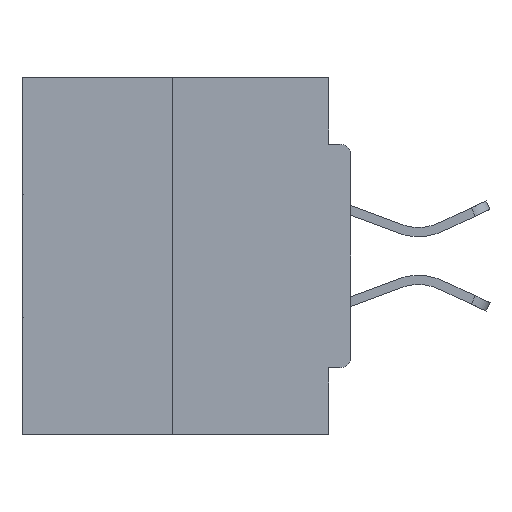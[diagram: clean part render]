
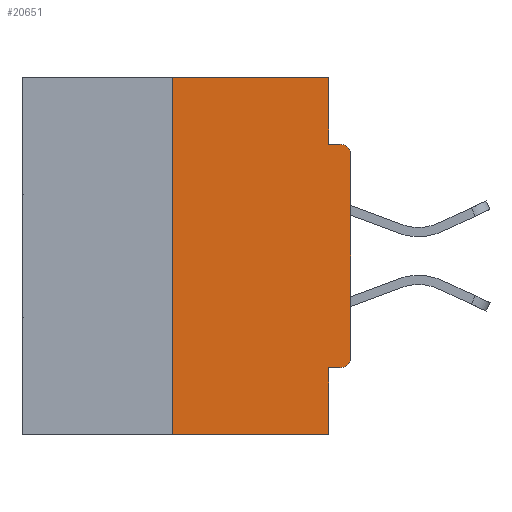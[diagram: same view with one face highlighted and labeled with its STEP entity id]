
A CAD part, left-side view. The second image highlights one B-rep face of the part: STEP entity #20651.
In plain terms, the highlighted planar face has unit normal (-1, 0, 0).
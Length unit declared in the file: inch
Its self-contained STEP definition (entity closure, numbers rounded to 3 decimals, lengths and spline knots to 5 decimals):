
#1036 = CARTESIAN_POINT ( 'NONE',  ( 0., 0., -0.0935 ) ) ;
#1229 = VERTEX_POINT ( 'NONE', #34514 ) ;
#1658 = VECTOR ( 'NONE', #26369, 39.37008 ) ;
#1724 = VECTOR ( 'NONE', #2325, 39.37008 ) ;
#2126 = ORIENTED_EDGE ( 'NONE', *, *, #22680, .F. ) ;
#2325 = DIRECTION ( 'NONE',  ( 0., 0., 1. ) ) ;
#2469 = EDGE_CURVE ( 'NONE', #12966, #9747, #3826, .T. ) ;
#2650 = PLANE ( 'NONE',  #9495 ) ;
#3304 = VERTEX_POINT ( 'NONE', #9077 ) ;
#3761 = CARTESIAN_POINT ( 'NONE',  ( 0., 0.031, -0.4065 ) ) ;
#3826 = LINE ( 'NONE', #34916, #12984 ) ;
#4241 = ORIENTED_EDGE ( 'NONE', *, *, #29061, .F. ) ;
#4413 = DIRECTION ( 'NONE',  ( 0., -1., 0. ) ) ;
#5447 = DIRECTION ( 'NONE',  ( 0., 0., -1. ) ) ;
#5550 = ORIENTED_EDGE ( 'NONE', *, *, #33950, .F. ) ;
#5840 = DIRECTION ( 'NONE',  ( 0., 0., -1. ) ) ;
#8347 = VECTOR ( 'NONE', #35288, 39.37008 ) ;
#8620 = CARTESIAN_POINT ( 'NONE',  ( 0., 0.46, 0. ) ) ;
#9013 = DIRECTION ( 'NONE',  ( 1., 0., 0. ) ) ;
#9077 = CARTESIAN_POINT ( 'NONE',  ( 0., 0.25, 0. ) ) ;
#9121 = ORIENTED_EDGE ( 'NONE', *, *, #2469, .T. ) ;
#9495 = AXIS2_PLACEMENT_3D ( 'NONE', #8620, #9013, #5447 ) ;
#9653 = VECTOR ( 'NONE', #19865, 39.37008 ) ;
#9747 = VERTEX_POINT ( 'NONE', #37930 ) ;
#10101 = DIRECTION ( 'NONE',  ( 0., -1., 0. ) ) ;
#10767 = CIRCLE ( 'NONE', #20283, 0.015 ) ;
#11812 = DIRECTION ( 'NONE',  ( -1., 0., 0. ) ) ;
#12966 = VERTEX_POINT ( 'NONE', #30072 ) ;
#12984 = VECTOR ( 'NONE', #4413, 39.37008 ) ;
#13275 = EDGE_CURVE ( 'NONE', #37519, #1229, #38341, .T. ) ;
#13367 = EDGE_CURVE ( 'NONE', #35274, #18704, #17462, .T. ) ;
#14390 = EDGE_CURVE ( 'NONE', #3304, #25434, #18477, .T. ) ;
#14423 = CARTESIAN_POINT ( 'NONE',  ( 0., 0.031, -0.5 ) ) ;
#14607 = VECTOR ( 'NONE', #37385, 39.37008 ) ;
#14666 = LINE ( 'NONE', #26224, #1724 ) ;
#15212 = CARTESIAN_POINT ( 'NONE',  ( 0., 0., -0.3915 ) ) ;
#15776 = EDGE_CURVE ( 'NONE', #27937, #37519, #14666, .T. ) ;
#16962 = LINE ( 'NONE', #24811, #14607 ) ;
#17132 = LINE ( 'NONE', #1036, #8347 ) ;
#17462 = LINE ( 'NONE', #26234, #27581 ) ;
#17970 = ORIENTED_EDGE ( 'NONE', *, *, #15776, .T. ) ;
#17973 = ORIENTED_EDGE ( 'NONE', *, *, #36122, .F. ) ;
#18477 = LINE ( 'NONE', #25251, #30253 ) ;
#18704 = VERTEX_POINT ( 'NONE', #3761 ) ;
#19720 = CARTESIAN_POINT ( 'NONE',  ( 0., 0., -0.1085 ) ) ;
#19865 = DIRECTION ( 'NONE',  ( 0., 0., 1. ) ) ;
#20283 = AXIS2_PLACEMENT_3D ( 'NONE', #26948, #11812, #5840 ) ;
#20390 = CARTESIAN_POINT ( 'NONE',  ( 0., 0.031, 0. ) ) ;
#20615 = EDGE_CURVE ( 'NONE', #35274, #27937, #10767, .T. ) ;
#20651 = ADVANCED_FACE ( 'NONE', ( #33340 ), #2650, .F. ) ;
#21119 = AXIS2_PLACEMENT_3D ( 'NONE', #36210, #35607, #33216 ) ;
#21245 = VERTEX_POINT ( 'NONE', #25091 ) ;
#22680 = EDGE_CURVE ( 'NONE', #21245, #1229, #17132, .T. ) ;
#23343 = ORIENTED_EDGE ( 'NONE', *, *, #20615, .T. ) ;
#23640 = ORIENTED_EDGE ( 'NONE', *, *, #13367, .F. ) ;
#24811 = CARTESIAN_POINT ( 'NONE',  ( 0., 0.031, 0. ) ) ;
#25091 = CARTESIAN_POINT ( 'NONE',  ( 0., 0.031, -0.0935 ) ) ;
#25251 = CARTESIAN_POINT ( 'NONE',  ( 0., 0.46, 0. ) ) ;
#25434 = VERTEX_POINT ( 'NONE', #20390 ) ;
#26224 = CARTESIAN_POINT ( 'NONE',  ( 0., 0., 0. ) ) ;
#26234 = CARTESIAN_POINT ( 'NONE',  ( 0., 0., -0.4065 ) ) ;
#26369 = DIRECTION ( 'NONE',  ( 0., 0., -1. ) ) ;
#26948 = CARTESIAN_POINT ( 'NONE',  ( 0., 0.015, -0.3915 ) ) ;
#27046 = ORIENTED_EDGE ( 'NONE', *, *, #14390, .F. ) ;
#27581 = VECTOR ( 'NONE', #32414, 39.37008 ) ;
#27937 = VERTEX_POINT ( 'NONE', #15212 ) ;
#29061 = EDGE_CURVE ( 'NONE', #18704, #9747, #38940, .T. ) ;
#30064 = EDGE_LOOP ( 'NONE', ( #27046, #17973, #9121, #4241, #23640, #23343, #17970, #39062, #2126, #5550 ) ) ;
#30072 = CARTESIAN_POINT ( 'NONE',  ( 0., 0.25, -0.5 ) ) ;
#30253 = VECTOR ( 'NONE', #10101, 39.37008 ) ;
#30995 = CARTESIAN_POINT ( 'NONE',  ( 0., 0.015, -0.4065 ) ) ;
#31830 = CARTESIAN_POINT ( 'NONE',  ( 0., 0.25, 0. ) ) ;
#32414 = DIRECTION ( 'NONE',  ( 0., 1., 0. ) ) ;
#33216 = DIRECTION ( 'NONE',  ( 0., 0., -1. ) ) ;
#33340 = FACE_OUTER_BOUND ( 'NONE', #30064, .T. ) ;
#33950 = EDGE_CURVE ( 'NONE', #25434, #21245, #16962, .T. ) ;
#34514 = CARTESIAN_POINT ( 'NONE',  ( 0., 0.015, -0.0935 ) ) ;
#34916 = CARTESIAN_POINT ( 'NONE',  ( 0., 0.46, -0.5 ) ) ;
#35028 = LINE ( 'NONE', #31830, #9653 ) ;
#35274 = VERTEX_POINT ( 'NONE', #30995 ) ;
#35288 = DIRECTION ( 'NONE',  ( 0., -1., 0. ) ) ;
#35607 = DIRECTION ( 'NONE',  ( -1., 0., 0. ) ) ;
#36122 = EDGE_CURVE ( 'NONE', #12966, #3304, #35028, .T. ) ;
#36210 = CARTESIAN_POINT ( 'NONE',  ( 0., 0.015, -0.1085 ) ) ;
#37385 = DIRECTION ( 'NONE',  ( 0., 0., -1. ) ) ;
#37519 = VERTEX_POINT ( 'NONE', #19720 ) ;
#37930 = CARTESIAN_POINT ( 'NONE',  ( 0., 0.031, -0.5 ) ) ;
#38341 = CIRCLE ( 'NONE', #21119, 0.015 ) ;
#38940 = LINE ( 'NONE', #14423, #1658 ) ;
#39062 = ORIENTED_EDGE ( 'NONE', *, *, #13275, .T. ) ;
